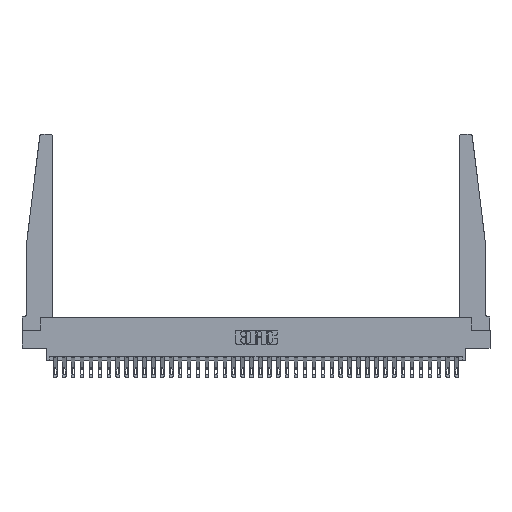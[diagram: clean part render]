
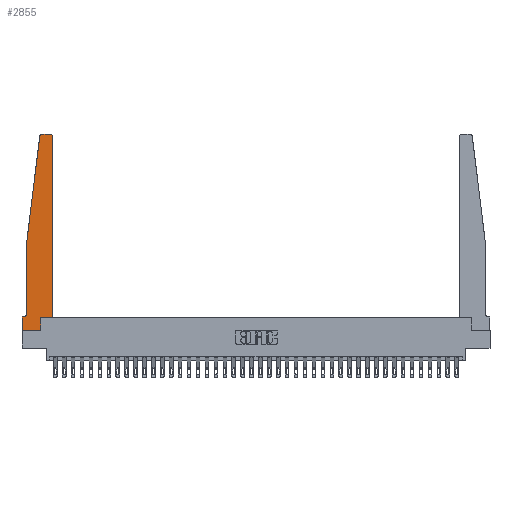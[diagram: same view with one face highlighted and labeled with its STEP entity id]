
A CAD part, top view. The second image highlights one B-rep face of the part: STEP entity #2855.
In plain terms, the highlighted planar face has unit normal (0, 0, 1).
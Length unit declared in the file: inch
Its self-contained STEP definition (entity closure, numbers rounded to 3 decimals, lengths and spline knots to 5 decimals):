
#529 = VERTEX_POINT ( 'NONE', #21944 ) ;
#746 = CARTESIAN_POINT ( 'NONE',  ( 0.015, 0.2375, 0.37 ) ) ;
#1125 = CARTESIAN_POINT ( 'NONE',  ( 0., 0., 0.37 ) ) ;
#1386 = VERTEX_POINT ( 'NONE', #29187 ) ;
#2100 = CARTESIAN_POINT ( 'NONE',  ( 0.065, 1.25, 0.37 ) ) ;
#2198 = ORIENTED_EDGE ( 'NONE', *, *, #8453, .T. ) ;
#2436 = ORIENTED_EDGE ( 'NONE', *, *, #29527, .T. ) ;
#2623 = LINE ( 'NONE', #27212, #13567 ) ;
#2855 = ADVANCED_FACE ( 'NONE', ( #19556 ), #27922, .T. ) ;
#3339 = DIRECTION ( 'NONE',  ( 0., 0., 1. ) ) ;
#3623 = VERTEX_POINT ( 'NONE', #7545 ) ;
#3884 = AXIS2_PLACEMENT_3D ( 'NONE', #26392, #31721, #7328 ) ;
#4346 = DIRECTION ( 'NONE',  ( 1., 0., 0. ) ) ;
#4988 = CARTESIAN_POINT ( 'NONE',  ( 0.2605, 0.18, 0.37 ) ) ;
#5028 = LINE ( 'NONE', #29272, #24928 ) ;
#5312 = VERTEX_POINT ( 'NONE', #33727 ) ;
#5380 = CARTESIAN_POINT ( 'NONE',  ( 0.24675, 2.72367, 0.37 ) ) ;
#5574 = CIRCLE ( 'NONE', #3884, 0.03 ) ;
#5987 = EDGE_CURVE ( 'NONE', #20306, #3623, #2623, .T. ) ;
#7117 = VERTEX_POINT ( 'NONE', #23344 ) ;
#7328 = DIRECTION ( 'NONE',  ( 1., 0., 0. ) ) ;
#7545 = CARTESIAN_POINT ( 'NONE',  ( 0., 0.1875, 0.37 ) ) ;
#8453 = EDGE_CURVE ( 'NONE', #1386, #18476, #29406, .T. ) ;
#8689 = CARTESIAN_POINT ( 'NONE',  ( 0., 0.1875, 0.37 ) ) ;
#9321 = CARTESIAN_POINT ( 'NONE',  ( 0.065, 1.25, 0.37 ) ) ;
#9426 = AXIS2_PLACEMENT_3D ( 'NONE', #25614, #18278, #26303 ) ;
#11222 = AXIS2_PLACEMENT_3D ( 'NONE', #8689, #3339, #14200 ) ;
#11868 = VECTOR ( 'NONE', #25238, 39.37008 ) ;
#12211 = VECTOR ( 'NONE', #17166, 39.37008 ) ;
#12325 = CARTESIAN_POINT ( 'NONE',  ( 0.015, 0.1875, 0.37 ) ) ;
#12491 = ORIENTED_EDGE ( 'NONE', *, *, #30885, .T. ) ;
#12718 = CARTESIAN_POINT ( 'NONE',  ( 0.425, 0.18, 0.37 ) ) ;
#13096 = CARTESIAN_POINT ( 'NONE',  ( 0.2605, 0.18, 0.37 ) ) ;
#13567 = VECTOR ( 'NONE', #13842, 39.37008 ) ;
#13842 = DIRECTION ( 'NONE',  ( -1., 0., 0. ) ) ;
#14200 = DIRECTION ( 'NONE',  ( 1., 0., 0. ) ) ;
#14313 = LINE ( 'NONE', #9321, #12211 ) ;
#15553 = DIRECTION ( 'NONE',  ( 0., 1., 0. ) ) ;
#15797 = VECTOR ( 'NONE', #16213, 39.37008 ) ;
#16166 = EDGE_CURVE ( 'NONE', #18063, #5312, #14313, .T. ) ;
#16213 = DIRECTION ( 'NONE',  ( 0., 1., 0. ) ) ;
#17166 = DIRECTION ( 'NONE',  ( 0., -1., 0. ) ) ;
#17208 = LINE ( 'NONE', #33756, #11868 ) ;
#17265 = VERTEX_POINT ( 'NONE', #5380 ) ;
#17301 = DIRECTION ( 'NONE',  ( 0., 0., -1. ) ) ;
#17364 = ORIENTED_EDGE ( 'NONE', *, *, #5987, .T. ) ;
#18063 = VERTEX_POINT ( 'NONE', #2100 ) ;
#18278 = DIRECTION ( 'NONE',  ( 0., 0., 1. ) ) ;
#18476 = VERTEX_POINT ( 'NONE', #13096 ) ;
#18523 = ORIENTED_EDGE ( 'NONE', *, *, #19547, .T. ) ;
#18534 = DIRECTION ( 'NONE',  ( -0.122, -0.992, 0. ) ) ;
#19547 = EDGE_CURVE ( 'NONE', #24523, #17265, #32733, .T. ) ;
#19556 = FACE_OUTER_BOUND ( 'NONE', #21178, .T. ) ;
#20306 = VERTEX_POINT ( 'NONE', #12325 ) ;
#20366 = VERTEX_POINT ( 'NONE', #1125 ) ;
#20678 = ORIENTED_EDGE ( 'NONE', *, *, #32171, .T. ) ;
#20853 = CARTESIAN_POINT ( 'NONE',  ( 0.065, 1.25, 0.37 ) ) ;
#20897 = CARTESIAN_POINT ( 'NONE',  ( 0.425, 0.18, 0.37 ) ) ;
#21178 = EDGE_LOOP ( 'NONE', ( #2436, #18523, #23802, #33626, #32628, #17364, #20678, #12491, #2198, #26138, #27015, #21650 ) ) ;
#21650 = ORIENTED_EDGE ( 'NONE', *, *, #29894, .T. ) ;
#21944 = CARTESIAN_POINT ( 'NONE',  ( 0.395, 2.75, 0.37 ) ) ;
#22684 = EDGE_CURVE ( 'NONE', #22904, #7117, #34405, .T. ) ;
#22904 = VERTEX_POINT ( 'NONE', #25341 ) ;
#23125 = EDGE_CURVE ( 'NONE', #17265, #18063, #24059, .T. ) ;
#23344 = CARTESIAN_POINT ( 'NONE',  ( 0.425, 2.72, 0.37 ) ) ;
#23802 = ORIENTED_EDGE ( 'NONE', *, *, #23125, .T. ) ;
#24059 = LINE ( 'NONE', #20853, #27808 ) ;
#24523 = VERTEX_POINT ( 'NONE', #26736 ) ;
#24928 = VECTOR ( 'NONE', #34586, 39.37008 ) ;
#24959 = VECTOR ( 'NONE', #15553, 39.37008 ) ;
#25238 = DIRECTION ( 'NONE',  ( 0., -1., 0. ) ) ;
#25341 = CARTESIAN_POINT ( 'NONE',  ( 0.425, 0.18, 0.37 ) ) ;
#25614 = CARTESIAN_POINT ( 'NONE',  ( 0.27653, 2.72, 0.37 ) ) ;
#26138 = ORIENTED_EDGE ( 'NONE', *, *, #31116, .T. ) ;
#26303 = DIRECTION ( 'NONE',  ( 1., 0., 0. ) ) ;
#26392 = CARTESIAN_POINT ( 'NONE',  ( 0.395, 2.72, 0.37 ) ) ;
#26736 = CARTESIAN_POINT ( 'NONE',  ( 0.27653, 2.75, 0.37 ) ) ;
#27015 = ORIENTED_EDGE ( 'NONE', *, *, #22684, .T. ) ;
#27212 = CARTESIAN_POINT ( 'NONE',  ( 0.065, 0.1875, 0.37 ) ) ;
#27232 = VECTOR ( 'NONE', #33576, 39.37008 ) ;
#27808 = VECTOR ( 'NONE', #18534, 39.37008 ) ;
#27922 = PLANE ( 'NONE',  #11222 ) ;
#27994 = DIRECTION ( 'NONE',  ( -1., 0., 0. ) ) ;
#28240 = LINE ( 'NONE', #33400, #27232 ) ;
#29187 = CARTESIAN_POINT ( 'NONE',  ( 0.2605, 0., 0.37 ) ) ;
#29272 = CARTESIAN_POINT ( 'NONE',  ( 0.25, 2.75, 0.37 ) ) ;
#29406 = LINE ( 'NONE', #4988, #15797 ) ;
#29527 = EDGE_CURVE ( 'NONE', #529, #24523, #5028, .T. ) ;
#29894 = EDGE_CURVE ( 'NONE', #7117, #529, #5574, .T. ) ;
#30112 = AXIS2_PLACEMENT_3D ( 'NONE', #746, #17301, #27994 ) ;
#30115 = VECTOR ( 'NONE', #4346, 39.37008 ) ;
#30885 = EDGE_CURVE ( 'NONE', #20366, #1386, #28240, .T. ) ;
#31116 = EDGE_CURVE ( 'NONE', #18476, #22904, #31589, .T. ) ;
#31241 = CIRCLE ( 'NONE', #30112, 0.05 ) ;
#31589 = LINE ( 'NONE', #12718, #30115 ) ;
#31721 = DIRECTION ( 'NONE',  ( 0., 0., 1. ) ) ;
#32171 = EDGE_CURVE ( 'NONE', #3623, #20366, #17208, .T. ) ;
#32628 = ORIENTED_EDGE ( 'NONE', *, *, #32997, .T. ) ;
#32733 = CIRCLE ( 'NONE', #9426, 0.03 ) ;
#32997 = EDGE_CURVE ( 'NONE', #5312, #20306, #31241, .T. ) ;
#33400 = CARTESIAN_POINT ( 'NONE',  ( 0., 0., 0.37 ) ) ;
#33576 = DIRECTION ( 'NONE',  ( 1., 0., 0. ) ) ;
#33626 = ORIENTED_EDGE ( 'NONE', *, *, #16166, .T. ) ;
#33727 = CARTESIAN_POINT ( 'NONE',  ( 0.065, 0.2375, 0.37 ) ) ;
#33756 = CARTESIAN_POINT ( 'NONE',  ( 0., 0., 0.37 ) ) ;
#34405 = LINE ( 'NONE', #20897, #24959 ) ;
#34586 = DIRECTION ( 'NONE',  ( -1., 0., 0. ) ) ;
